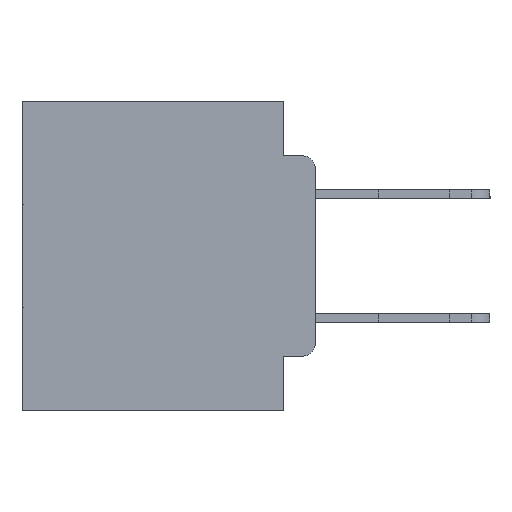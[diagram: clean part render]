
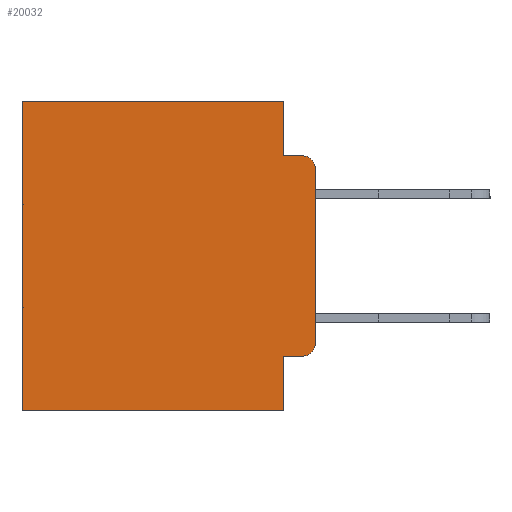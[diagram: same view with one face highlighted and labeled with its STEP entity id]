
A CAD part, left-side view. The second image highlights one B-rep face of the part: STEP entity #20032.
In plain terms, the highlighted planar face has unit normal (-1, 0, 0).
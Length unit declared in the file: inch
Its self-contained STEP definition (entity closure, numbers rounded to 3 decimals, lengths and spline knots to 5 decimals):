
#586 = CARTESIAN_POINT ( 'NONE',  ( 0.298, 0., -0.1085 ) ) ;
#649 = VECTOR ( 'NONE', #26211, 39.37008 ) ;
#749 = LINE ( 'NONE', #12537, #13056 ) ;
#954 = EDGE_CURVE ( 'NONE', #25972, #18953, #22028, .T. ) ;
#1058 = LINE ( 'NONE', #29366, #6567 ) ;
#1073 = DIRECTION ( 'NONE',  ( 0., 0., -1. ) ) ;
#1428 = VERTEX_POINT ( 'NONE', #19309 ) ;
#1932 = LINE ( 'NONE', #26743, #19669 ) ;
#2470 = CARTESIAN_POINT ( 'NONE',  ( 0.298, 0.02, -0.4115 ) ) ;
#2515 = EDGE_CURVE ( 'NONE', #4414, #18953, #22274, .T. ) ;
#2572 = ORIENTED_EDGE ( 'NONE', *, *, #954, .F. ) ;
#3076 = CARTESIAN_POINT ( 'NONE',  ( 0.298, 0.051, 0. ) ) ;
#4408 = CARTESIAN_POINT ( 'NONE',  ( 0.298, 0., 0. ) ) ;
#4414 = VERTEX_POINT ( 'NONE', #586 ) ;
#4485 = ORIENTED_EDGE ( 'NONE', *, *, #18582, .T. ) ;
#5024 = VERTEX_POINT ( 'NONE', #19293 ) ;
#5128 = AXIS2_PLACEMENT_3D ( 'NONE', #13950, #13683, #1073 ) ;
#6089 = VERTEX_POINT ( 'NONE', #2470 ) ;
#6328 = ORIENTED_EDGE ( 'NONE', *, *, #26624, .F. ) ;
#6567 = VECTOR ( 'NONE', #27130, 39.37008 ) ;
#6580 = VERTEX_POINT ( 'NONE', #3076 ) ;
#7046 = DIRECTION ( 'NONE',  ( 1., 0., 0. ) ) ;
#7920 = VECTOR ( 'NONE', #23668, 39.37008 ) ;
#8256 = DIRECTION ( 'NONE',  ( 0., -1., 0. ) ) ;
#8331 = LINE ( 'NONE', #4408, #19078 ) ;
#8964 = AXIS2_PLACEMENT_3D ( 'NONE', #13812, #7046, #23147 ) ;
#9719 = DIRECTION ( 'NONE',  ( 0., -1., 0. ) ) ;
#9788 = CARTESIAN_POINT ( 'NONE',  ( 0.298, 0.02, -0.0885 ) ) ;
#10248 = AXIS2_PLACEMENT_3D ( 'NONE', #26725, #12975, #28967 ) ;
#10294 = EDGE_CURVE ( 'NONE', #4414, #5024, #8331, .T. ) ;
#10473 = ORIENTED_EDGE ( 'NONE', *, *, #23250, .F. ) ;
#12474 = CARTESIAN_POINT ( 'NONE',  ( 0.298, 0.051, -0.0885 ) ) ;
#12537 = CARTESIAN_POINT ( 'NONE',  ( 0.298, 0., -0.5 ) ) ;
#12945 = LINE ( 'NONE', #14664, #649 ) ;
#12975 = DIRECTION ( 'NONE',  ( -1., 0., 0. ) ) ;
#13056 = VECTOR ( 'NONE', #26388, 39.37008 ) ;
#13215 = LINE ( 'NONE', #21361, #7920 ) ;
#13559 = DIRECTION ( 'NONE',  ( 0., 0., -1. ) ) ;
#13683 = DIRECTION ( 'NONE',  ( -1., 0., 0. ) ) ;
#13812 = CARTESIAN_POINT ( 'NONE',  ( 0.298, 0., 0. ) ) ;
#13950 = CARTESIAN_POINT ( 'NONE',  ( 0.298, 0.02, -0.1085 ) ) ;
#13973 = EDGE_LOOP ( 'NONE', ( #25569, #19008, #2572, #25486, #18117, #15696, #6328, #10473, #19110, #4485 ) ) ;
#14090 = VERTEX_POINT ( 'NONE', #15032 ) ;
#14664 = CARTESIAN_POINT ( 'NONE',  ( 0.298, 0.051, 0. ) ) ;
#14920 = FACE_OUTER_BOUND ( 'NONE', #13973, .T. ) ;
#15032 = CARTESIAN_POINT ( 'NONE',  ( 0.298, 0.051, -0.4115 ) ) ;
#15112 = VECTOR ( 'NONE', #8256, 39.37008 ) ;
#15696 = ORIENTED_EDGE ( 'NONE', *, *, #24757, .T. ) ;
#18117 = ORIENTED_EDGE ( 'NONE', *, *, #25509, .T. ) ;
#18582 = EDGE_CURVE ( 'NONE', #6089, #5024, #27450, .T. ) ;
#18873 = CARTESIAN_POINT ( 'NONE',  ( 0.298, 0.051, -0.4115 ) ) ;
#18953 = VERTEX_POINT ( 'NONE', #9788 ) ;
#19008 = ORIENTED_EDGE ( 'NONE', *, *, #2515, .T. ) ;
#19078 = VECTOR ( 'NONE', #13559, 39.37008 ) ;
#19110 = ORIENTED_EDGE ( 'NONE', *, *, #20139, .T. ) ;
#19293 = CARTESIAN_POINT ( 'NONE',  ( 0.298, 0., -0.3915 ) ) ;
#19309 = CARTESIAN_POINT ( 'NONE',  ( 0.298, 0.473, -0.5 ) ) ;
#19669 = VECTOR ( 'NONE', #28891, 39.37008 ) ;
#19867 = VERTEX_POINT ( 'NONE', #22549 ) ;
#20032 = ADVANCED_FACE ( 'NONE', ( #14920 ), #20826, .F. ) ;
#20139 = EDGE_CURVE ( 'NONE', #14090, #6089, #29518, .T. ) ;
#20826 = PLANE ( 'NONE',  #8964 ) ;
#21361 = CARTESIAN_POINT ( 'NONE',  ( 0.298, 0.473, 0. ) ) ;
#22028 = LINE ( 'NONE', #27231, #15112 ) ;
#22274 = CIRCLE ( 'NONE', #5128, 0.02 ) ;
#22549 = CARTESIAN_POINT ( 'NONE',  ( 0.298, 0.051, -0.5 ) ) ;
#23147 = DIRECTION ( 'NONE',  ( 0., 0., -1. ) ) ;
#23250 = EDGE_CURVE ( 'NONE', #14090, #19867, #12945, .T. ) ;
#23607 = VECTOR ( 'NONE', #9719, 39.37008 ) ;
#23668 = DIRECTION ( 'NONE',  ( 0., 0., -1. ) ) ;
#24757 = EDGE_CURVE ( 'NONE', #26754, #1428, #13215, .T. ) ;
#25486 = ORIENTED_EDGE ( 'NONE', *, *, #27734, .F. ) ;
#25509 = EDGE_CURVE ( 'NONE', #6580, #26754, #1932, .T. ) ;
#25569 = ORIENTED_EDGE ( 'NONE', *, *, #10294, .F. ) ;
#25917 = CARTESIAN_POINT ( 'NONE',  ( 0.298, 0.473, 0. ) ) ;
#25972 = VERTEX_POINT ( 'NONE', #12474 ) ;
#26211 = DIRECTION ( 'NONE',  ( 0., 0., -1. ) ) ;
#26388 = DIRECTION ( 'NONE',  ( 0., 1., 0. ) ) ;
#26624 = EDGE_CURVE ( 'NONE', #19867, #1428, #749, .T. ) ;
#26725 = CARTESIAN_POINT ( 'NONE',  ( 0.298, 0.02, -0.3915 ) ) ;
#26743 = CARTESIAN_POINT ( 'NONE',  ( 0.298, 0., 0. ) ) ;
#26754 = VERTEX_POINT ( 'NONE', #25917 ) ;
#27130 = DIRECTION ( 'NONE',  ( 0., 0., -1. ) ) ;
#27231 = CARTESIAN_POINT ( 'NONE',  ( 0.298, 0.051, -0.0885 ) ) ;
#27450 = CIRCLE ( 'NONE', #10248, 0.02 ) ;
#27734 = EDGE_CURVE ( 'NONE', #6580, #25972, #1058, .T. ) ;
#28891 = DIRECTION ( 'NONE',  ( 0., 1., 0. ) ) ;
#28967 = DIRECTION ( 'NONE',  ( 0., 0., -1. ) ) ;
#29366 = CARTESIAN_POINT ( 'NONE',  ( 0.298, 0.051, 0. ) ) ;
#29518 = LINE ( 'NONE', #18873, #23607 ) ;
